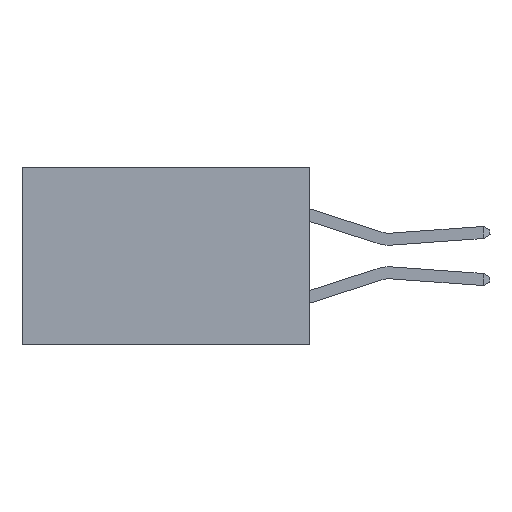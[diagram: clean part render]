
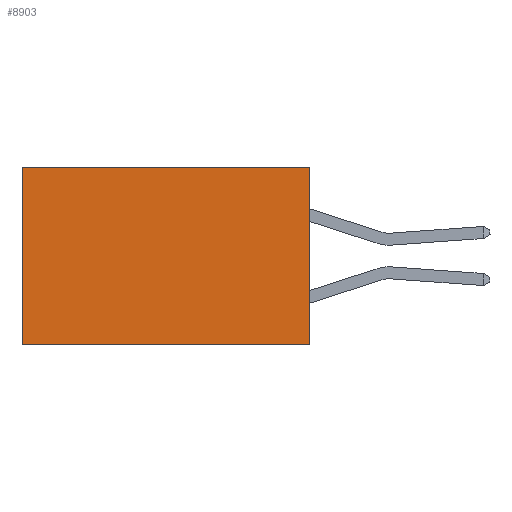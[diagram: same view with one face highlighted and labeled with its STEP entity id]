
A CAD part, left-side view. The second image highlights one B-rep face of the part: STEP entity #8903.
In plain terms, the highlighted planar face has unit normal (-1, 0, 0).
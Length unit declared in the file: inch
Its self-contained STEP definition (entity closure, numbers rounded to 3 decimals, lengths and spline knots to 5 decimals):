
#423 = VECTOR ( 'NONE', #4984, 39.37008 ) ;
#818 = DIRECTION ( 'NONE',  ( 0., 0., -1. ) ) ;
#1176 = DIRECTION ( 'NONE',  ( 0., 0., -1. ) ) ;
#1412 = LINE ( 'NONE', #5841, #423 ) ;
#1454 = EDGE_LOOP ( 'NONE', ( #2986, #2465, #6402, #9423 ) ) ;
#1518 = VECTOR ( 'NONE', #4163, 39.37008 ) ;
#2149 = FACE_OUTER_BOUND ( 'NONE', #1454, .T. ) ;
#2443 = CARTESIAN_POINT ( 'NONE',  ( 0.2615, 0., -0.37 ) ) ;
#2465 = ORIENTED_EDGE ( 'NONE', *, *, #6867, .F. ) ;
#2493 = CARTESIAN_POINT ( 'NONE',  ( 0.2615, 0.6, -0.37 ) ) ;
#2925 = VERTEX_POINT ( 'NONE', #3984 ) ;
#2986 = ORIENTED_EDGE ( 'NONE', *, *, #8621, .T. ) ;
#3035 = CARTESIAN_POINT ( 'NONE',  ( 0.2615, 0., -0.37 ) ) ;
#3174 = LINE ( 'NONE', #2443, #1518 ) ;
#3984 = CARTESIAN_POINT ( 'NONE',  ( 0.2615, 0., -0.37 ) ) ;
#4163 = DIRECTION ( 'NONE',  ( 0., 1., 0. ) ) ;
#4457 = LINE ( 'NONE', #5310, #10498 ) ;
#4940 = CARTESIAN_POINT ( 'NONE',  ( 0.2615, 0., 0. ) ) ;
#4984 = DIRECTION ( 'NONE',  ( 0., 1., 0. ) ) ;
#5051 = AXIS2_PLACEMENT_3D ( 'NONE', #3035, #9779, #5667 ) ;
#5310 = CARTESIAN_POINT ( 'NONE',  ( 0.2615, 0., -0.37 ) ) ;
#5667 = DIRECTION ( 'NONE',  ( 0., 0., -1. ) ) ;
#5841 = CARTESIAN_POINT ( 'NONE',  ( 0.2615, 0., 0. ) ) ;
#6060 = VERTEX_POINT ( 'NONE', #4940 ) ;
#6121 = CARTESIAN_POINT ( 'NONE',  ( 0.2615, 0.6, 0. ) ) ;
#6402 = ORIENTED_EDGE ( 'NONE', *, *, #9718, .F. ) ;
#6827 = VECTOR ( 'NONE', #818, 39.37008 ) ;
#6867 = EDGE_CURVE ( 'NONE', #2925, #10618, #3174, .T. ) ;
#7548 = LINE ( 'NONE', #2493, #6827 ) ;
#7874 = PLANE ( 'NONE',  #5051 ) ;
#8621 = EDGE_CURVE ( 'NONE', #10707, #10618, #7548, .T. ) ;
#8903 = ADVANCED_FACE ( 'NONE', ( #2149 ), #7874, .F. ) ;
#8919 = EDGE_CURVE ( 'NONE', #6060, #10707, #1412, .T. ) ;
#9423 = ORIENTED_EDGE ( 'NONE', *, *, #8919, .T. ) ;
#9718 = EDGE_CURVE ( 'NONE', #6060, #2925, #4457, .T. ) ;
#9779 = DIRECTION ( 'NONE',  ( 1., 0., 0. ) ) ;
#10442 = CARTESIAN_POINT ( 'NONE',  ( 0.2615, 0.6, -0.37 ) ) ;
#10498 = VECTOR ( 'NONE', #1176, 39.37008 ) ;
#10618 = VERTEX_POINT ( 'NONE', #10442 ) ;
#10707 = VERTEX_POINT ( 'NONE', #6121 ) ;
